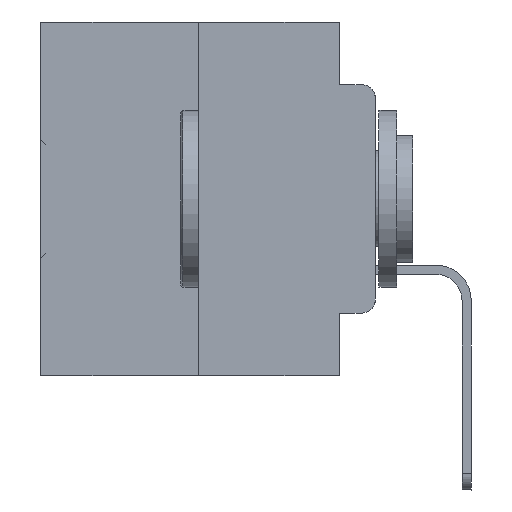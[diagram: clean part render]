
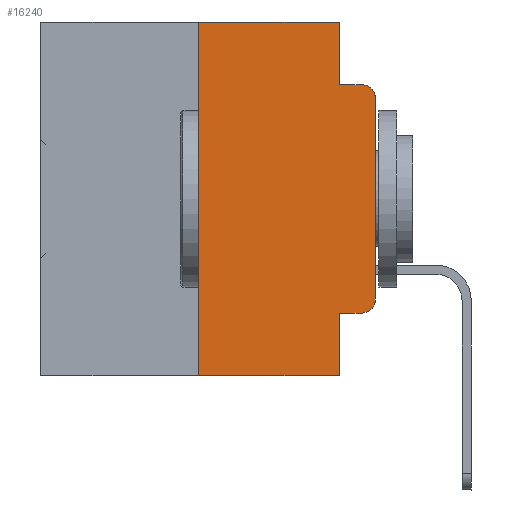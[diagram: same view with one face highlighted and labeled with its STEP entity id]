
A CAD part, left-side view. The second image highlights one B-rep face of the part: STEP entity #16240.
In plain terms, the highlighted planar face has unit normal (-1, 0, 0).
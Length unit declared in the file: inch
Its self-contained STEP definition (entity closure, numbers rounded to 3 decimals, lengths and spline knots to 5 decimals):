
#626 = ORIENTED_EDGE ( 'NONE', *, *, #8226, .T. ) ;
#973 = VECTOR ( 'NONE', #16511, 39.37008 ) ;
#1133 = ORIENTED_EDGE ( 'NONE', *, *, #20869, .T. ) ;
#1159 = CARTESIAN_POINT ( 'NONE',  ( 0., 0.051, -0.5 ) ) ;
#1675 = EDGE_CURVE ( 'NONE', #3470, #17532, #2221, .T. ) ;
#2221 = LINE ( 'NONE', #11828, #3878 ) ;
#2313 = AXIS2_PLACEMENT_3D ( 'NONE', #25642, #31278, #23313 ) ;
#2515 = CARTESIAN_POINT ( 'NONE',  ( 0., 0.051, 0. ) ) ;
#2690 = ORIENTED_EDGE ( 'NONE', *, *, #22908, .T. ) ;
#3013 = VECTOR ( 'NONE', #4483, 39.37008 ) ;
#3151 = ORIENTED_EDGE ( 'NONE', *, *, #32010, .F. ) ;
#3190 = DIRECTION ( 'NONE',  ( 0., -1., 0. ) ) ;
#3470 = VERTEX_POINT ( 'NONE', #14590 ) ;
#3855 = LINE ( 'NONE', #28170, #3013 ) ;
#3878 = VECTOR ( 'NONE', #9306, 39.37008 ) ;
#4095 = DIRECTION ( 'NONE',  ( -1., 0., 0. ) ) ;
#4130 = DIRECTION ( 'NONE',  ( 0., 0., -1. ) ) ;
#4483 = DIRECTION ( 'NONE',  ( 0., -1., 0. ) ) ;
#4695 = CARTESIAN_POINT ( 'NONE',  ( 0., 0.25, 0. ) ) ;
#4805 = CARTESIAN_POINT ( 'NONE',  ( 0., 0.051, -0.4115 ) ) ;
#4974 = VECTOR ( 'NONE', #31205, 39.37008 ) ;
#5369 = EDGE_CURVE ( 'NONE', #32734, #17532, #16444, .T. ) ;
#5414 = DIRECTION ( 'NONE',  ( 1., 0., 0. ) ) ;
#5495 = VERTEX_POINT ( 'NONE', #4695 ) ;
#5532 = PLANE ( 'NONE',  #11701 ) ;
#5633 = VERTEX_POINT ( 'NONE', #8266 ) ;
#5854 = DIRECTION ( 'NONE',  ( 0., 0., -1. ) ) ;
#8058 = ORIENTED_EDGE ( 'NONE', *, *, #5369, .F. ) ;
#8226 = EDGE_CURVE ( 'NONE', #13723, #25381, #17361, .T. ) ;
#8266 = CARTESIAN_POINT ( 'NONE',  ( 0., 0.02, -0.4115 ) ) ;
#8351 = FACE_OUTER_BOUND ( 'NONE', #28676, .T. ) ;
#8484 = CIRCLE ( 'NONE', #2313, 0.02 ) ;
#8750 = VECTOR ( 'NONE', #3190, 39.37008 ) ;
#8910 = CARTESIAN_POINT ( 'NONE',  ( 0., 0.051, -0.0885 ) ) ;
#8943 = VERTEX_POINT ( 'NONE', #31584 ) ;
#9306 = DIRECTION ( 'NONE',  ( 0., -1., 0. ) ) ;
#11701 = AXIS2_PLACEMENT_3D ( 'NONE', #27019, #5414, #5854 ) ;
#11740 = DIRECTION ( 'NONE',  ( 0., 0., 1. ) ) ;
#11828 = CARTESIAN_POINT ( 'NONE',  ( 0., 0.473, -0.5 ) ) ;
#11900 = ORIENTED_EDGE ( 'NONE', *, *, #28844, .F. ) ;
#11943 = VECTOR ( 'NONE', #21789, 39.37008 ) ;
#12568 = AXIS2_PLACEMENT_3D ( 'NONE', #30436, #4095, #33353 ) ;
#12762 = LINE ( 'NONE', #16434, #11943 ) ;
#12848 = LINE ( 'NONE', #13657, #8750 ) ;
#12852 = LINE ( 'NONE', #16823, #13679 ) ;
#13137 = ORIENTED_EDGE ( 'NONE', *, *, #15794, .F. ) ;
#13657 = CARTESIAN_POINT ( 'NONE',  ( 0., 0.051, -0.4115 ) ) ;
#13679 = VECTOR ( 'NONE', #11740, 39.37008 ) ;
#13723 = VERTEX_POINT ( 'NONE', #26908 ) ;
#14405 = CARTESIAN_POINT ( 'NONE',  ( 0., 0.051, -0.0885 ) ) ;
#14590 = CARTESIAN_POINT ( 'NONE',  ( 0., 0.25, -0.5 ) ) ;
#15794 = EDGE_CURVE ( 'NONE', #24202, #8943, #24542, .T. ) ;
#16240 = ADVANCED_FACE ( 'NONE', ( #8351 ), #5532, .F. ) ;
#16434 = CARTESIAN_POINT ( 'NONE',  ( 0., 0.051, 0. ) ) ;
#16444 = LINE ( 'NONE', #30929, #28860 ) ;
#16511 = DIRECTION ( 'NONE',  ( 0., -1., 0. ) ) ;
#16823 = CARTESIAN_POINT ( 'NONE',  ( 0., 0.25, 0. ) ) ;
#17114 = ORIENTED_EDGE ( 'NONE', *, *, #32522, .F. ) ;
#17361 = LINE ( 'NONE', #17793, #4974 ) ;
#17532 = VERTEX_POINT ( 'NONE', #1159 ) ;
#17793 = CARTESIAN_POINT ( 'NONE',  ( 0., 0., 0. ) ) ;
#20869 = EDGE_CURVE ( 'NONE', #5633, #13723, #8484, .T. ) ;
#21205 = ORIENTED_EDGE ( 'NONE', *, *, #23690, .T. ) ;
#21789 = DIRECTION ( 'NONE',  ( 0., 0., -1. ) ) ;
#22017 = CARTESIAN_POINT ( 'NONE',  ( 0., 0., -0.1085 ) ) ;
#22908 = EDGE_CURVE ( 'NONE', #32734, #5633, #12848, .T. ) ;
#23313 = DIRECTION ( 'NONE',  ( 0., 0., -1. ) ) ;
#23690 = EDGE_CURVE ( 'NONE', #25381, #8943, #33916, .T. ) ;
#24202 = VERTEX_POINT ( 'NONE', #14405 ) ;
#24542 = LINE ( 'NONE', #8910, #973 ) ;
#25381 = VERTEX_POINT ( 'NONE', #22017 ) ;
#25642 = CARTESIAN_POINT ( 'NONE',  ( 0., 0.02, -0.3915 ) ) ;
#26908 = CARTESIAN_POINT ( 'NONE',  ( 0., 0., -0.3915 ) ) ;
#27019 = CARTESIAN_POINT ( 'NONE',  ( 0., 0.473, 0. ) ) ;
#28030 = ORIENTED_EDGE ( 'NONE', *, *, #1675, .T. ) ;
#28170 = CARTESIAN_POINT ( 'NONE',  ( 0., 0.473, 0. ) ) ;
#28676 = EDGE_LOOP ( 'NONE', ( #626, #21205, #13137, #11900, #3151, #17114, #28030, #8058, #2690, #1133 ) ) ;
#28844 = EDGE_CURVE ( 'NONE', #34151, #24202, #12762, .T. ) ;
#28860 = VECTOR ( 'NONE', #4130, 39.37008 ) ;
#30436 = CARTESIAN_POINT ( 'NONE',  ( 0., 0.02, -0.1085 ) ) ;
#30929 = CARTESIAN_POINT ( 'NONE',  ( 0., 0.051, 0. ) ) ;
#31205 = DIRECTION ( 'NONE',  ( 0., 0., 1. ) ) ;
#31278 = DIRECTION ( 'NONE',  ( -1., 0., 0. ) ) ;
#31584 = CARTESIAN_POINT ( 'NONE',  ( 0., 0.02, -0.0885 ) ) ;
#32010 = EDGE_CURVE ( 'NONE', #5495, #34151, #3855, .T. ) ;
#32522 = EDGE_CURVE ( 'NONE', #3470, #5495, #12852, .T. ) ;
#32734 = VERTEX_POINT ( 'NONE', #4805 ) ;
#33353 = DIRECTION ( 'NONE',  ( 0., 0., -1. ) ) ;
#33916 = CIRCLE ( 'NONE', #12568, 0.02 ) ;
#34151 = VERTEX_POINT ( 'NONE', #2515 ) ;
